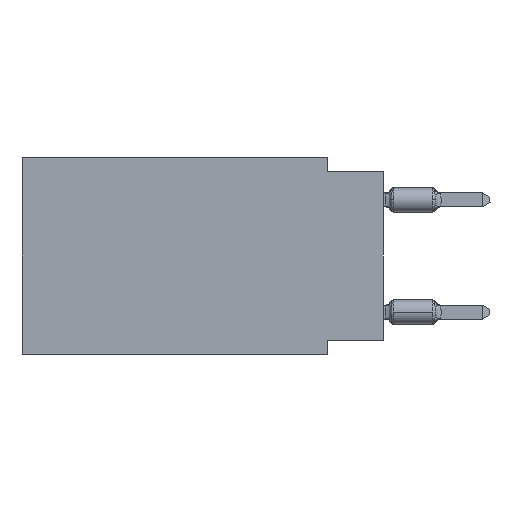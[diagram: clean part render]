
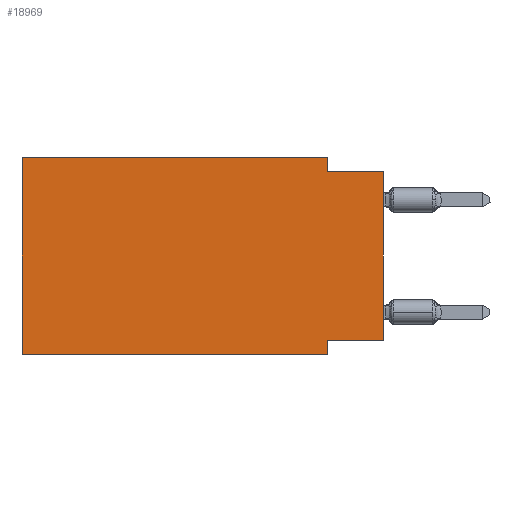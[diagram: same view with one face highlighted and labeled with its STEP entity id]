
A CAD part, left-side view. The second image highlights one B-rep face of the part: STEP entity #18969.
In plain terms, the highlighted planar face has unit normal (-1, 0, 0).
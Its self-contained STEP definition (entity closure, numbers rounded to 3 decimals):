
#403 = VERTEX_POINT ( 'NONE', #4021 ) ;
#554 = ORIENTED_EDGE ( 'NONE', *, *, #12657, .F. ) ;
#3114 = CARTESIAN_POINT ( 'NONE',  ( 0., 2.54, -8.255 ) ) ;
#3736 = DIRECTION ( 'NONE',  ( 0., 0., -1. ) ) ;
#3839 = VERTEX_POINT ( 'NONE', #9015 ) ;
#3916 = CARTESIAN_POINT ( 'NONE',  ( 0., 16.383, 0. ) ) ;
#3995 = PLANE ( 'NONE',  #15560 ) ;
#4021 = CARTESIAN_POINT ( 'NONE',  ( 0., 16.383, 0. ) ) ;
#4146 = LINE ( 'NONE', #3916, #20888 ) ;
#4188 = VERTEX_POINT ( 'NONE', #19389 ) ;
#4301 = VECTOR ( 'NONE', #10412, 1000. ) ;
#5151 = EDGE_CURVE ( 'NONE', #4188, #3839, #16741, .T. ) ;
#5222 = VERTEX_POINT ( 'NONE', #5567 ) ;
#5563 = ORIENTED_EDGE ( 'NONE', *, *, #11972, .T. ) ;
#5567 = CARTESIAN_POINT ( 'NONE',  ( 0., 2.54, 0. ) ) ;
#5658 = DIRECTION ( 'NONE',  ( 0., -1., 0. ) ) ;
#5854 = CARTESIAN_POINT ( 'NONE',  ( 0., 0., -8.255 ) ) ;
#5883 = DIRECTION ( 'NONE',  ( 1., 0., 0. ) ) ;
#6086 = LINE ( 'NONE', #5854, #13841 ) ;
#6987 = VERTEX_POINT ( 'NONE', #20175 ) ;
#7551 = LINE ( 'NONE', #22996, #17482 ) ;
#9015 = CARTESIAN_POINT ( 'NONE',  ( 0., 2.54, -8.89 ) ) ;
#9435 = ORIENTED_EDGE ( 'NONE', *, *, #23427, .F. ) ;
#9669 = FACE_OUTER_BOUND ( 'NONE', #16938, .T. ) ;
#9999 = ORIENTED_EDGE ( 'NONE', *, *, #20895, .F. ) ;
#10382 = CARTESIAN_POINT ( 'NONE',  ( 0., 0., 0. ) ) ;
#10390 = LINE ( 'NONE', #19513, #18289 ) ;
#10412 = DIRECTION ( 'NONE',  ( 0., -1., 0. ) ) ;
#10526 = DIRECTION ( 'NONE',  ( 0., -1., 0. ) ) ;
#10693 = VECTOR ( 'NONE', #21000, 1000. ) ;
#11028 = VERTEX_POINT ( 'NONE', #23789 ) ;
#11464 = ORIENTED_EDGE ( 'NONE', *, *, #15885, .F. ) ;
#11779 = DIRECTION ( 'NONE',  ( 0., 0., -1. ) ) ;
#11925 = LINE ( 'NONE', #19659, #4301 ) ;
#11972 = EDGE_CURVE ( 'NONE', #11028, #12641, #16194, .T. ) ;
#12159 = ORIENTED_EDGE ( 'NONE', *, *, #18190, .F. ) ;
#12441 = CARTESIAN_POINT ( 'NONE',  ( 0., 16.383, -8.89 ) ) ;
#12641 = VERTEX_POINT ( 'NONE', #13509 ) ;
#12652 = VECTOR ( 'NONE', #10526, 1000. ) ;
#12657 = EDGE_CURVE ( 'NONE', #4188, #403, #4146, .T. ) ;
#13509 = CARTESIAN_POINT ( 'NONE',  ( 0., 0., -0.635 ) ) ;
#13521 = ORIENTED_EDGE ( 'NONE', *, *, #16592, .F. ) ;
#13639 = DIRECTION ( 'NONE',  ( 0., 0., 1. ) ) ;
#13841 = VECTOR ( 'NONE', #15699, 1000. ) ;
#15040 = CARTESIAN_POINT ( 'NONE',  ( 0., 2.54, -8.89 ) ) ;
#15229 = ORIENTED_EDGE ( 'NONE', *, *, #5151, .T. ) ;
#15560 = AXIS2_PLACEMENT_3D ( 'NONE', #19299, #5883, #3736 ) ;
#15665 = VERTEX_POINT ( 'NONE', #3114 ) ;
#15699 = DIRECTION ( 'NONE',  ( 0., 1., 0. ) ) ;
#15885 = EDGE_CURVE ( 'NONE', #5222, #6987, #10390, .T. ) ;
#16194 = LINE ( 'NONE', #10382, #18851 ) ;
#16592 = EDGE_CURVE ( 'NONE', #403, #5222, #7551, .T. ) ;
#16741 = LINE ( 'NONE', #12441, #12652 ) ;
#16938 = EDGE_LOOP ( 'NONE', ( #5563, #9435, #11464, #13521, #554, #15229, #12159, #9999 ) ) ;
#17482 = VECTOR ( 'NONE', #5658, 1000. ) ;
#18190 = EDGE_CURVE ( 'NONE', #15665, #3839, #24428, .T. ) ;
#18289 = VECTOR ( 'NONE', #11779, 1000. ) ;
#18851 = VECTOR ( 'NONE', #23818, 1000. ) ;
#18969 = ADVANCED_FACE ( 'NONE', ( #9669 ), #3995, .F. ) ;
#19299 = CARTESIAN_POINT ( 'NONE',  ( 0., 16.383, 0. ) ) ;
#19389 = CARTESIAN_POINT ( 'NONE',  ( 0., 16.383, -8.89 ) ) ;
#19513 = CARTESIAN_POINT ( 'NONE',  ( 0., 2.54, 0. ) ) ;
#19659 = CARTESIAN_POINT ( 'NONE',  ( 0., 0., -0.635 ) ) ;
#20175 = CARTESIAN_POINT ( 'NONE',  ( 0., 2.54, -0.635 ) ) ;
#20888 = VECTOR ( 'NONE', #13639, 1000. ) ;
#20895 = EDGE_CURVE ( 'NONE', #11028, #15665, #6086, .T. ) ;
#21000 = DIRECTION ( 'NONE',  ( 0., 0., -1. ) ) ;
#22996 = CARTESIAN_POINT ( 'NONE',  ( 0., 16.383, 0. ) ) ;
#23427 = EDGE_CURVE ( 'NONE', #6987, #12641, #11925, .T. ) ;
#23789 = CARTESIAN_POINT ( 'NONE',  ( 0., 0., -8.255 ) ) ;
#23818 = DIRECTION ( 'NONE',  ( 0., 0., 1. ) ) ;
#24428 = LINE ( 'NONE', #15040, #10693 ) ;
